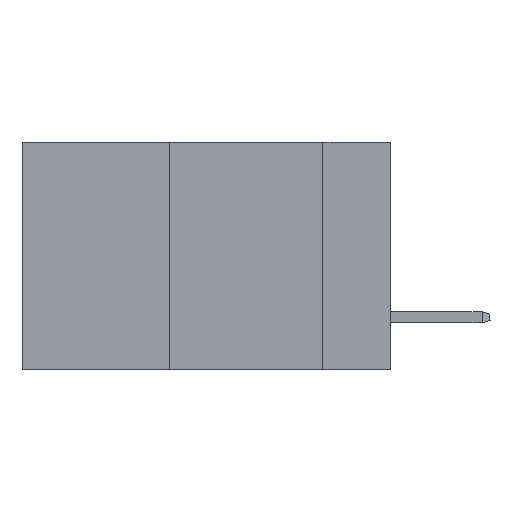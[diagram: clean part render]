
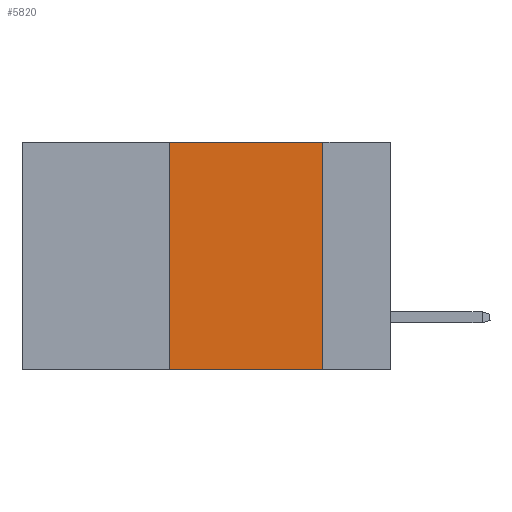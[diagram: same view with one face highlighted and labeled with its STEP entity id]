
A CAD part, left-side view. The second image highlights one B-rep face of the part: STEP entity #5820.
In plain terms, the highlighted planar face has unit normal (-1, 0, 0).
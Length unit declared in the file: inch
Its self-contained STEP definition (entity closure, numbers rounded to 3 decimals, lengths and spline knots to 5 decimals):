
#1256 = LINE ( 'NONE', #8546, #18026 ) ;
#1301 = EDGE_CURVE ( 'NONE', #15567, #7961, #1522, .T. ) ;
#1375 = VERTEX_POINT ( 'NONE', #14062 ) ;
#1419 = AXIS2_PLACEMENT_3D ( 'NONE', #18113, #16205, #12880 ) ;
#1426 = CARTESIAN_POINT ( 'NONE',  ( 0., 0.36, 0. ) ) ;
#1522 = LINE ( 'NONE', #7128, #22028 ) ;
#1641 = VECTOR ( 'NONE', #5009, 39.37008 ) ;
#1722 = ORIENTED_EDGE ( 'NONE', *, *, #20001, .F. ) ;
#2307 = LINE ( 'NONE', #11027, #8084 ) ;
#3067 = ORIENTED_EDGE ( 'NONE', *, *, #19666, .F. ) ;
#3107 = LINE ( 'NONE', #1426, #1641 ) ;
#3406 = CARTESIAN_POINT ( 'NONE',  ( 0., 0.11, -0.37 ) ) ;
#3592 = VERTEX_POINT ( 'NONE', #13887 ) ;
#4104 = ORIENTED_EDGE ( 'NONE', *, *, #1301, .T. ) ;
#5009 = DIRECTION ( 'NONE',  ( 0., 0., 1. ) ) ;
#5278 = EDGE_LOOP ( 'NONE', ( #1722, #12980, #3067, #4104 ) ) ;
#5820 = ADVANCED_FACE ( 'NONE', ( #8934 ), #21934, .F. ) ;
#6902 = DIRECTION ( 'NONE',  ( 0., -1., 0. ) ) ;
#7081 = CARTESIAN_POINT ( 'NONE',  ( 0., 0.36, -0.37 ) ) ;
#7128 = CARTESIAN_POINT ( 'NONE',  ( 0., 0.6, -0.37 ) ) ;
#7961 = VERTEX_POINT ( 'NONE', #3406 ) ;
#8084 = VECTOR ( 'NONE', #9593, 39.37008 ) ;
#8546 = CARTESIAN_POINT ( 'NONE',  ( 0., 0.11, 0. ) ) ;
#8934 = FACE_OUTER_BOUND ( 'NONE', #5278, .T. ) ;
#9593 = DIRECTION ( 'NONE',  ( 0., -1., 0. ) ) ;
#11027 = CARTESIAN_POINT ( 'NONE',  ( 0., 0.6, 0. ) ) ;
#12880 = DIRECTION ( 'NONE',  ( 0., 0., -1. ) ) ;
#12980 = ORIENTED_EDGE ( 'NONE', *, *, #16987, .F. ) ;
#13887 = CARTESIAN_POINT ( 'NONE',  ( 0., 0.11, 0. ) ) ;
#14062 = CARTESIAN_POINT ( 'NONE',  ( 0., 0.36, 0. ) ) ;
#15567 = VERTEX_POINT ( 'NONE', #7081 ) ;
#15821 = DIRECTION ( 'NONE',  ( 0., 0., -1. ) ) ;
#16205 = DIRECTION ( 'NONE',  ( 1., 0., 0. ) ) ;
#16987 = EDGE_CURVE ( 'NONE', #1375, #3592, #2307, .T. ) ;
#18026 = VECTOR ( 'NONE', #15821, 39.37008 ) ;
#18113 = CARTESIAN_POINT ( 'NONE',  ( 0., 0.6, 0. ) ) ;
#19666 = EDGE_CURVE ( 'NONE', #15567, #1375, #3107, .T. ) ;
#20001 = EDGE_CURVE ( 'NONE', #3592, #7961, #1256, .T. ) ;
#21934 = PLANE ( 'NONE',  #1419 ) ;
#22028 = VECTOR ( 'NONE', #6902, 39.37008 ) ;
